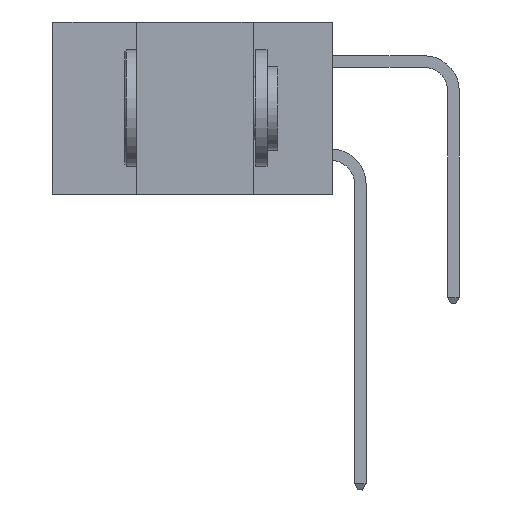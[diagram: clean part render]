
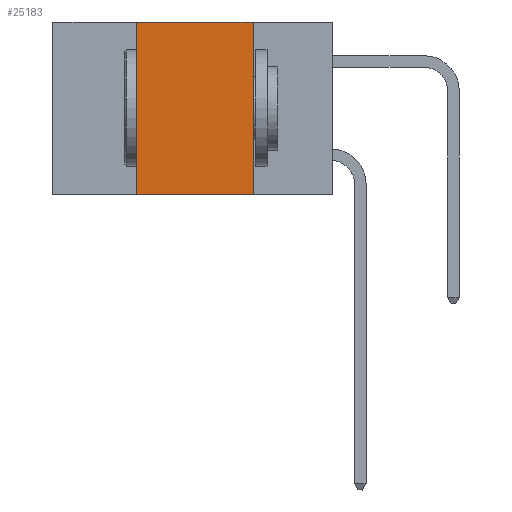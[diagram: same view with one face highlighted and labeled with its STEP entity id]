
A CAD part, left-side view. The second image highlights one B-rep face of the part: STEP entity #25183.
In plain terms, the highlighted planar face has unit normal (-1, 0, 0).
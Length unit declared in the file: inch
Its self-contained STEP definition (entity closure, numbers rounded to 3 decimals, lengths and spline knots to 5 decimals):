
#1134 = DIRECTION ( 'NONE',  ( 0., -1., 0. ) ) ;
#4134 = VECTOR ( 'NONE', #1134, 39.37008 ) ;
#5457 = EDGE_CURVE ( 'NONE', #12804, #19878, #22874, .T. ) ;
#6824 = ORIENTED_EDGE ( 'NONE', *, *, #21949, .F. ) ;
#8167 = VERTEX_POINT ( 'NONE', #35639 ) ;
#8692 = CARTESIAN_POINT ( 'NONE',  ( 0., 0.6, 0. ) ) ;
#9320 = VECTOR ( 'NONE', #31309, 39.37008 ) ;
#9323 = DIRECTION ( 'NONE',  ( 0., 0., 1. ) ) ;
#9327 = CARTESIAN_POINT ( 'NONE',  ( 0., 0.17, 0. ) ) ;
#10177 = LINE ( 'NONE', #9327, #9320 ) ;
#12202 = EDGE_LOOP ( 'NONE', ( #21143, #6824, #31032, #28525 ) ) ;
#12804 = VERTEX_POINT ( 'NONE', #19237 ) ;
#13180 = CARTESIAN_POINT ( 'NONE',  ( 0., 0.17, -0.37 ) ) ;
#14257 = VECTOR ( 'NONE', #9323, 39.37008 ) ;
#14287 = PLANE ( 'NONE',  #35035 ) ;
#15104 = CARTESIAN_POINT ( 'NONE',  ( 0., 0.42, 0. ) ) ;
#16225 = EDGE_CURVE ( 'NONE', #8167, #19878, #10177, .T. ) ;
#16798 = VERTEX_POINT ( 'NONE', #15104 ) ;
#17068 = DIRECTION ( 'NONE',  ( 0., 0., -1. ) ) ;
#19237 = CARTESIAN_POINT ( 'NONE',  ( 0., 0.42, -0.37 ) ) ;
#19878 = VERTEX_POINT ( 'NONE', #13180 ) ;
#20708 = LINE ( 'NONE', #23071, #14257 ) ;
#21143 = ORIENTED_EDGE ( 'NONE', *, *, #16225, .F. ) ;
#21949 = EDGE_CURVE ( 'NONE', #16798, #8167, #26199, .T. ) ;
#22874 = LINE ( 'NONE', #33552, #29276 ) ;
#23071 = CARTESIAN_POINT ( 'NONE',  ( 0., 0.42, 0. ) ) ;
#25183 = ADVANCED_FACE ( 'NONE', ( #31209 ), #14287, .F. ) ;
#26199 = LINE ( 'NONE', #34217, #4134 ) ;
#28485 = DIRECTION ( 'NONE',  ( 0., -1., 0. ) ) ;
#28525 = ORIENTED_EDGE ( 'NONE', *, *, #5457, .T. ) ;
#29276 = VECTOR ( 'NONE', #28485, 39.37008 ) ;
#31032 = ORIENTED_EDGE ( 'NONE', *, *, #31335, .F. ) ;
#31209 = FACE_OUTER_BOUND ( 'NONE', #12202, .T. ) ;
#31309 = DIRECTION ( 'NONE',  ( 0., 0., -1. ) ) ;
#31335 = EDGE_CURVE ( 'NONE', #12804, #16798, #20708, .T. ) ;
#33420 = DIRECTION ( 'NONE',  ( 1., 0., 0. ) ) ;
#33552 = CARTESIAN_POINT ( 'NONE',  ( 0., 0.6, -0.37 ) ) ;
#34217 = CARTESIAN_POINT ( 'NONE',  ( 0., 0.6, 0. ) ) ;
#35035 = AXIS2_PLACEMENT_3D ( 'NONE', #8692, #33420, #17068 ) ;
#35639 = CARTESIAN_POINT ( 'NONE',  ( 0., 0.17, 0. ) ) ;
